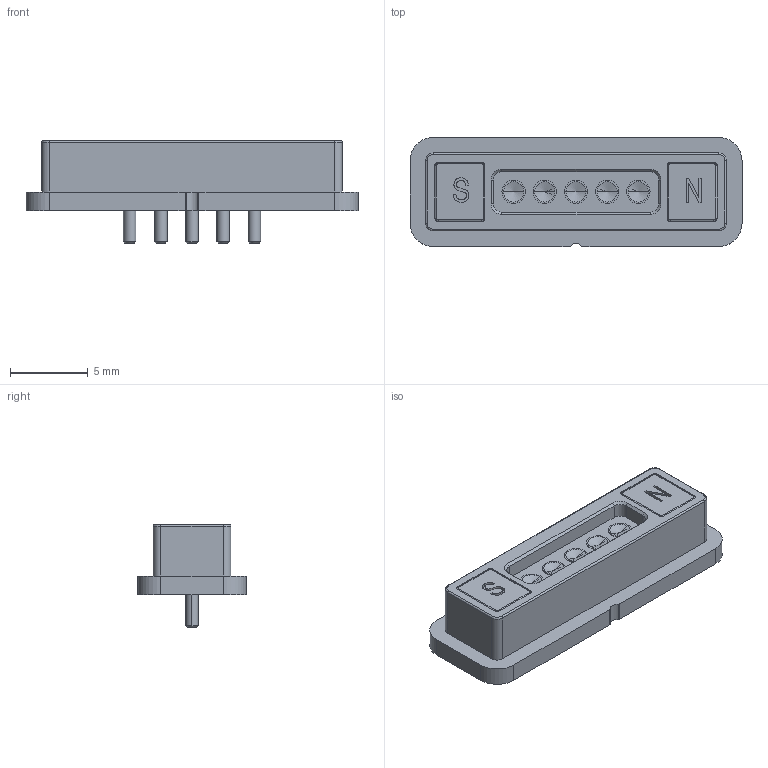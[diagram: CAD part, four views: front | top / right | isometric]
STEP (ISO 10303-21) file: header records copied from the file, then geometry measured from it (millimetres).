
FILE_DESCRIPTION (( 'STEP AP203' ), '1' );
FILE_NAME ('686-J0521250110.STEP', '2023-02-14T11:58:19', ( 'Magnum' ), ( '' ), 'SwSTEP 2.0', 'SolidWorks 2020', '' );
FILE_SCHEMA (( 'CONFIG_CONTROL_DESIGN' ));
Length unit declared in the file: millimetre
Products named in the file (1): 686-J0521250110
Bounding box: 21.3 x 7 x 6.6 mm (x, y, z)
Volume: 430.8 mm3; surface area: 691 mm2
Topology: 6 solids, 8 shells, 236 faces, 558 edges, 348 vertices
Faces by surface type: plane 90, cylinder 81, cone 31, bspline 20, torus 14
Entity records: 7582 total; most frequent: CARTESIAN_POINT 2053, DIRECTION 1171, ORIENTED_EDGE 1096, EDGE_CURVE 548, AXIS2_PLACEMENT_3D 434, VERTEX_POINT 348, LINE 303, VECTOR 303
